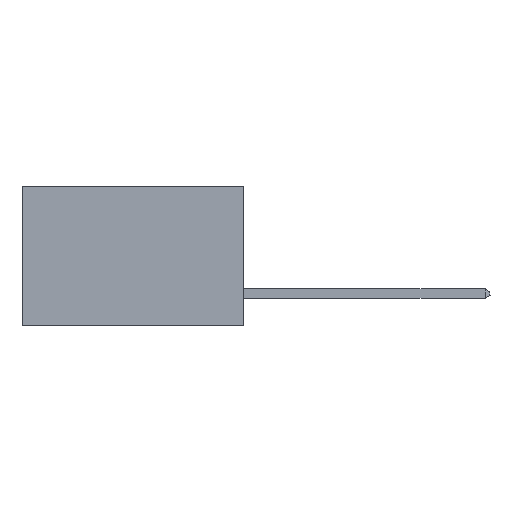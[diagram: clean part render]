
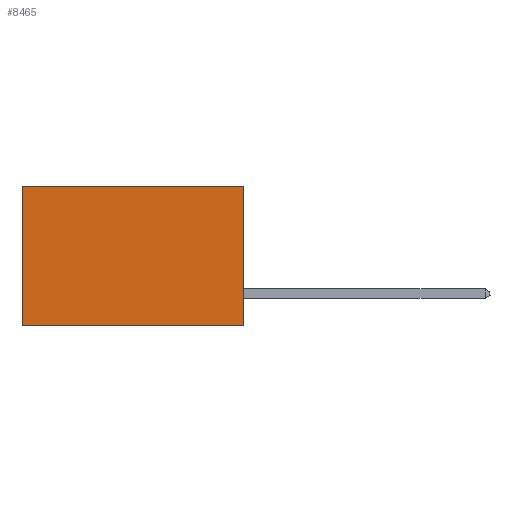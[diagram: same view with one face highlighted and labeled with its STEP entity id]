
A CAD part, left-side view. The second image highlights one B-rep face of the part: STEP entity #8465.
In plain terms, the highlighted planar face has unit normal (-1, 0, 0).
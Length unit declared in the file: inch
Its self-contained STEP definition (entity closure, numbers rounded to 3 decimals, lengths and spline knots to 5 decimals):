
#17 = LINE ( 'NONE', #10830, #8349 ) ;
#99 = ORIENTED_EDGE ( 'NONE', *, *, #4341, .T. ) ;
#155 = ORIENTED_EDGE ( 'NONE', *, *, #1742, .F. ) ;
#165 = ORIENTED_EDGE ( 'NONE', *, *, #1761, .F. ) ;
#188 = ORIENTED_EDGE ( 'NONE', *, *, #3400, .T. ) ;
#782 = VERTEX_POINT ( 'NONE', #11947 ) ;
#1144 = DIRECTION ( 'NONE',  ( 0., 0., -1. ) ) ;
#1157 = CARTESIAN_POINT ( 'NONE',  ( 0.277, 0., -0.37 ) ) ;
#1742 = EDGE_CURVE ( 'NONE', #12582, #782, #10514, .T. ) ;
#1761 = EDGE_CURVE ( 'NONE', #6353, #12582, #5180, .T. ) ;
#1773 = VECTOR ( 'NONE', #6939, 39.37008 ) ;
#1812 = CARTESIAN_POINT ( 'NONE',  ( 0.277, 0., 0. ) ) ;
#2462 = DIRECTION ( 'NONE',  ( 0., 1., 0. ) ) ;
#2540 = VECTOR ( 'NONE', #4375, 39.37008 ) ;
#3253 = CARTESIAN_POINT ( 'NONE',  ( 0.277, 0., -0.37 ) ) ;
#3400 = EDGE_CURVE ( 'NONE', #6353, #8589, #17, .T. ) ;
#3531 = DIRECTION ( 'NONE',  ( 0., 0., -1. ) ) ;
#4341 = EDGE_CURVE ( 'NONE', #8589, #782, #12307, .T. ) ;
#4375 = DIRECTION ( 'NONE',  ( 0., 1., 0. ) ) ;
#5180 = LINE ( 'NONE', #12208, #12053 ) ;
#6353 = VERTEX_POINT ( 'NONE', #1812 ) ;
#6939 = DIRECTION ( 'NONE',  ( 0., 0., -1. ) ) ;
#7032 = CARTESIAN_POINT ( 'NONE',  ( 0.277, 0.59, -0.37 ) ) ;
#8349 = VECTOR ( 'NONE', #2462, 39.37008 ) ;
#8465 = ADVANCED_FACE ( 'NONE', ( #11225 ), #8554, .F. ) ;
#8554 = PLANE ( 'NONE',  #13092 ) ;
#8589 = VERTEX_POINT ( 'NONE', #11424 ) ;
#8959 = EDGE_LOOP ( 'NONE', ( #99, #155, #165, #188 ) ) ;
#9482 = DIRECTION ( 'NONE',  ( 1., 0., 0. ) ) ;
#9827 = CARTESIAN_POINT ( 'NONE',  ( 0.277, 0., -0.37 ) ) ;
#10514 = LINE ( 'NONE', #9827, #2540 ) ;
#10830 = CARTESIAN_POINT ( 'NONE',  ( 0.277, 0., 0. ) ) ;
#11225 = FACE_OUTER_BOUND ( 'NONE', #8959, .T. ) ;
#11424 = CARTESIAN_POINT ( 'NONE',  ( 0.277, 0.59, 0. ) ) ;
#11947 = CARTESIAN_POINT ( 'NONE',  ( 0.277, 0.59, -0.37 ) ) ;
#12053 = VECTOR ( 'NONE', #1144, 39.37008 ) ;
#12208 = CARTESIAN_POINT ( 'NONE',  ( 0.277, 0., -0.37 ) ) ;
#12307 = LINE ( 'NONE', #7032, #1773 ) ;
#12582 = VERTEX_POINT ( 'NONE', #3253 ) ;
#13092 = AXIS2_PLACEMENT_3D ( 'NONE', #1157, #9482, #3531 ) ;
